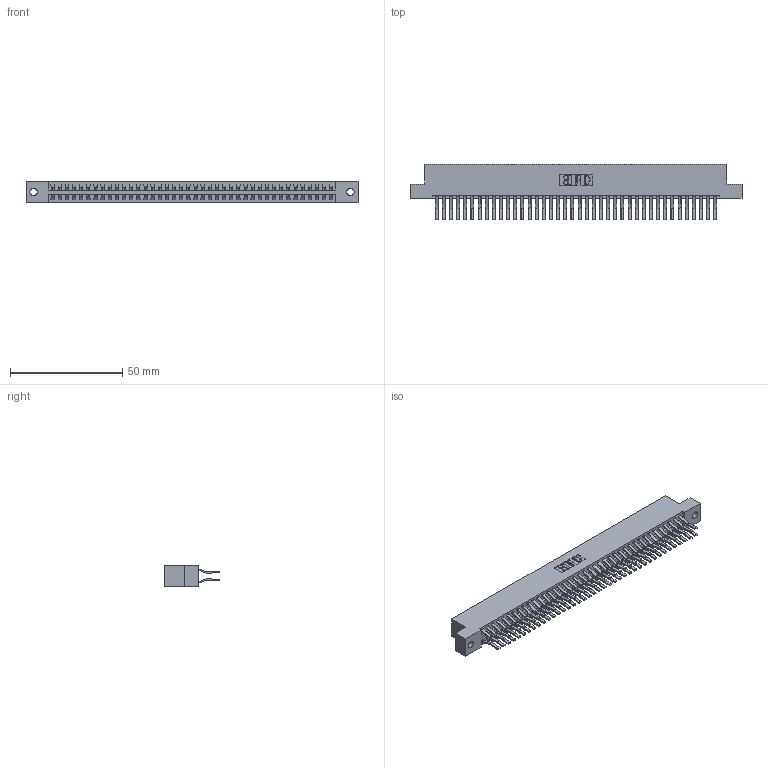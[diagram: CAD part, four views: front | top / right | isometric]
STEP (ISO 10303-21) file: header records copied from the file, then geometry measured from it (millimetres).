
FILE_DESCRIPTION (( 'STEP AP203' ), '1' );
FILE_NAME ('396-080-560-202.STEP', '2018-09-09T21:55:28', ( '' ), ( '' ), 'SwSTEP 2.0', 'SolidWorks 2016', '' );
FILE_SCHEMA (( 'CONFIG_CONTROL_DESIGN' ));
Length unit declared in the file: inch
Products named in the file (3): 345-292-001_560 Tail; 396-080-560-202; 346 Part_Flush Mounting Lugs - 0.128 Dia
Assembly tree (81 placements, depth 2):
  396-080-560-202
    346 Part_Flush Mounting Lugs - 0.128 Dia
    345-292-001_560 Tail  x80
Bounding box: 147.57 x 24.78 x 9.4 mm (x, y, z)
Volume: 14862.5 mm3; surface area: 21527.7 mm2
Topology: 81 solids, 81 shells, 4442 faces, 13209 edges, 8698 vertices
Faces by surface type: plane 2876, cylinder 1566
Entity records: 26465 total; most frequent: CARTESIAN_POINT 4364, ORIENTED_EDGE 4298, DIRECTION 3901, EDGE_CURVE 2149, VECTOR 1853, LINE 1853, VERTEX_POINT 1430, AXIS2_PLACEMENT_3D 1024
